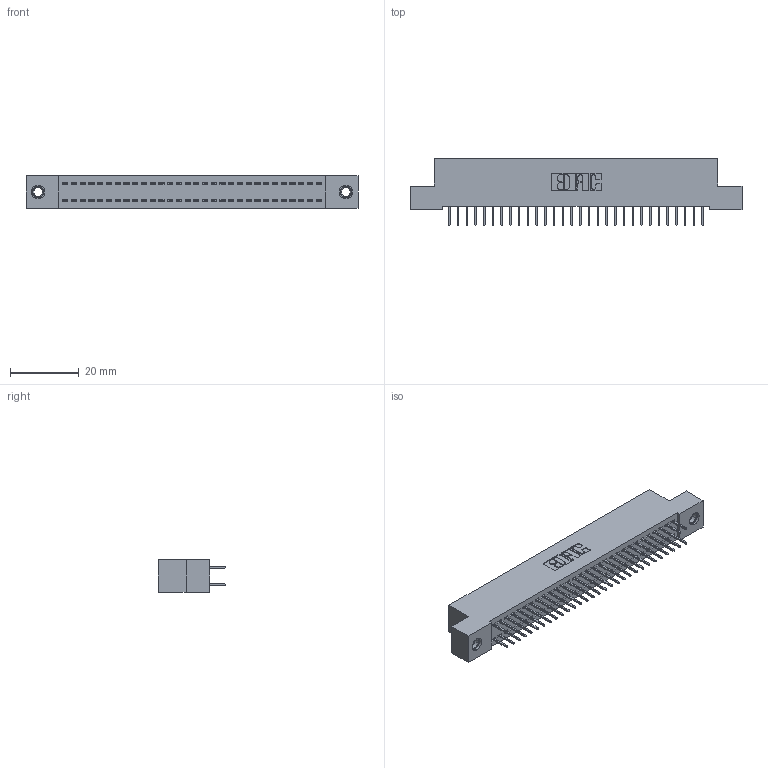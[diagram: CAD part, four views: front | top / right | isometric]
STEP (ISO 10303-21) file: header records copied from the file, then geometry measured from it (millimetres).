
FILE_DESCRIPTION (( 'STEP AP203' ), '1' );
FILE_NAME ('392-060-524-207.STEP', '2018-08-17T19:11:16', ( '' ), ( '' ), 'SwSTEP 2.0', 'SolidWorks 2016', '' );
FILE_SCHEMA (( 'CONFIG_CONTROL_DESIGN' ));
Length unit declared in the file: inch
Products named in the file (4): 392-060-524-207; 342 Part_TI; 345-292-001_345-293-124; 345-250-001_345-250-005-103
Assembly tree (63 placements, depth 2):
  392-060-524-207
    342 Part_TI
    345-292-001_345-293-124  x60
    345-250-001_345-250-005-103  x2
Bounding box: 96.52 x 19.69 x 9.4 mm (x, y, z)
Volume: 8512 mm3; surface area: 13349.4 mm2
Topology: 63 solids, 63 shells, 3530 faces, 9975 edges, 6402 vertices
Faces by surface type: plane 2618, cylinder 896, cone 12, torus 4
Entity records: 21980 total; most frequent: CARTESIAN_POINT 3637, ORIENTED_EDGE 3566, DIRECTION 3161, EDGE_CURVE 1783, VECTOR 1639, LINE 1639, VERTEX_POINT 1180, AXIS2_PLACEMENT_3D 761
